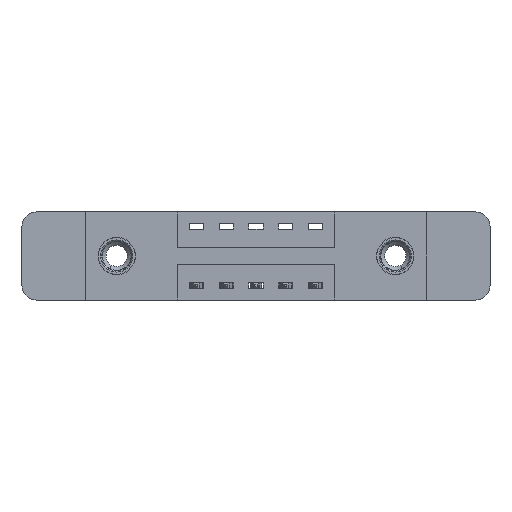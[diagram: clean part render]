
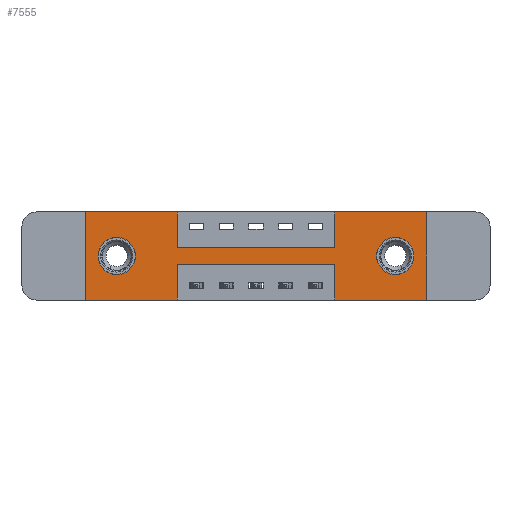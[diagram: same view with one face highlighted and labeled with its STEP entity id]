
A CAD part, front view. The second image highlights one B-rep face of the part: STEP entity #7555.
In plain terms, the highlighted planar face has unit normal (0, -1, 0).
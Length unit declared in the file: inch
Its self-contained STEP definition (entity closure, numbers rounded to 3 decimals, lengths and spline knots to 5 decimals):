
#7 = EDGE_CURVE ( 'NONE', #7786, #2454, #1814, .T. ) ;
#80 = CARTESIAN_POINT ( 'NONE',  ( 0.3875, 0., -0.15 ) ) ;
#185 = EDGE_CURVE ( 'NONE', #9656, #5307, #685, .T. ) ;
#569 = DIRECTION ( 'NONE',  ( 0., 0., -1. ) ) ;
#576 = CARTESIAN_POINT ( 'NONE',  ( 1.435, 0., -0.37 ) ) ;
#598 = DIRECTION ( 'NONE',  ( 1., 0., 0. ) ) ;
#685 = CIRCLE ( 'NONE', #3351, 0.078 ) ;
#688 = CARTESIAN_POINT ( 'NONE',  ( 1.3025, 0., -0.107 ) ) ;
#735 = CARTESIAN_POINT ( 'NONE',  ( 1.0475, 0., -0.15 ) ) ;
#748 = EDGE_CURVE ( 'NONE', #1055, #12500, #4042, .T. ) ;
#827 = EDGE_CURVE ( 'NONE', #8503, #7786, #8581, .T. ) ;
#932 = ORIENTED_EDGE ( 'NONE', *, *, #4530, .F. ) ;
#994 = CARTESIAN_POINT ( 'NONE',  ( 0., 0., 0. ) ) ;
#1055 = VERTEX_POINT ( 'NONE', #735 ) ;
#1070 = EDGE_LOOP ( 'NONE', ( #12165, #3451 ) ) ;
#1083 = EDGE_CURVE ( 'NONE', #12500, #12833, #3960, .T. ) ;
#1120 = CARTESIAN_POINT ( 'NONE',  ( 1.3025, 0., -0.185 ) ) ;
#1148 = DIRECTION ( 'NONE',  ( -1., 0., 0. ) ) ;
#1228 = VERTEX_POINT ( 'NONE', #576 ) ;
#1241 = ORIENTED_EDGE ( 'NONE', *, *, #9918, .F. ) ;
#1318 = CARTESIAN_POINT ( 'NONE',  ( 0.3875, 0., 0. ) ) ;
#1526 = EDGE_CURVE ( 'NONE', #2454, #10739, #7697, .T. ) ;
#1574 = DIRECTION ( 'NONE',  ( 0., 0., 1. ) ) ;
#1666 = FACE_BOUND ( 'NONE', #1070, .T. ) ;
#1814 = LINE ( 'NONE', #994, #6678 ) ;
#1844 = VECTOR ( 'NONE', #8648, 39.37008 ) ;
#1869 = CARTESIAN_POINT ( 'NONE',  ( 1.0475, 0., 0. ) ) ;
#1933 = EDGE_CURVE ( 'NONE', #12833, #1228, #7547, .T. ) ;
#1997 = CARTESIAN_POINT ( 'NONE',  ( 0.1325, 0., -0.263 ) ) ;
#2264 = DIRECTION ( 'NONE',  ( 0., 0., -1. ) ) ;
#2392 = EDGE_CURVE ( 'NONE', #12311, #5553, #10341, .T. ) ;
#2421 = EDGE_CURVE ( 'NONE', #5553, #12311, #3495, .T. ) ;
#2454 = VERTEX_POINT ( 'NONE', #4477 ) ;
#2648 = CARTESIAN_POINT ( 'NONE',  ( 0.3875, 0., -0.37 ) ) ;
#2805 = DIRECTION ( 'NONE',  ( 0., 0., -1. ) ) ;
#2867 = DIRECTION ( 'NONE',  ( 0., 0., 1. ) ) ;
#3082 = DIRECTION ( 'NONE',  ( 0., 0., -1. ) ) ;
#3159 = CARTESIAN_POINT ( 'NONE',  ( 1.3025, 0., -0.263 ) ) ;
#3272 = VERTEX_POINT ( 'NONE', #5117 ) ;
#3351 = AXIS2_PLACEMENT_3D ( 'NONE', #8488, #3353, #7647 ) ;
#3353 = DIRECTION ( 'NONE',  ( 0., 1., 0. ) ) ;
#3428 = DIRECTION ( 'NONE',  ( 0., 0., -1. ) ) ;
#3451 = ORIENTED_EDGE ( 'NONE', *, *, #12681, .T. ) ;
#3495 = CIRCLE ( 'NONE', #12816, 0.078 ) ;
#3581 = ORIENTED_EDGE ( 'NONE', *, *, #1933, .F. ) ;
#3729 = VERTEX_POINT ( 'NONE', #5995 ) ;
#3768 = FACE_BOUND ( 'NONE', #7127, .T. ) ;
#3927 = CARTESIAN_POINT ( 'NONE',  ( 0.1325, 0., -0.107 ) ) ;
#3960 = LINE ( 'NONE', #6140, #5457 ) ;
#3982 = ORIENTED_EDGE ( 'NONE', *, *, #748, .F. ) ;
#4029 = DIRECTION ( 'NONE',  ( -1., 0., 0. ) ) ;
#4042 = LINE ( 'NONE', #10263, #10501 ) ;
#4073 = DIRECTION ( 'NONE',  ( 1., 0., 0. ) ) ;
#4165 = CARTESIAN_POINT ( 'NONE',  ( 1.435, 0., 0. ) ) ;
#4201 = DIRECTION ( 'NONE',  ( 0., 0., -1. ) ) ;
#4278 = EDGE_CURVE ( 'NONE', #3729, #3272, #6508, .T. ) ;
#4341 = AXIS2_PLACEMENT_3D ( 'NONE', #12305, #9233, #2805 ) ;
#4477 = CARTESIAN_POINT ( 'NONE',  ( 0.3875, 0., 0. ) ) ;
#4530 = EDGE_CURVE ( 'NONE', #1228, #3729, #12153, .T. ) ;
#5050 = VECTOR ( 'NONE', #3428, 39.37008 ) ;
#5063 = DIRECTION ( 'NONE',  ( 0., 1., 0. ) ) ;
#5117 = CARTESIAN_POINT ( 'NONE',  ( 1.0475, 0., -0.22 ) ) ;
#5216 = EDGE_LOOP ( 'NONE', ( #11760, #1241, #5515, #932, #3581, #10585, #3982, #10959, #8956, #6202, #7494, #9322 ) ) ;
#5307 = VERTEX_POINT ( 'NONE', #1997 ) ;
#5457 = VECTOR ( 'NONE', #598, 39.37008 ) ;
#5515 = ORIENTED_EDGE ( 'NONE', *, *, #4278, .F. ) ;
#5553 = VERTEX_POINT ( 'NONE', #3159 ) ;
#5995 = CARTESIAN_POINT ( 'NONE',  ( 1.0475, 0., -0.37 ) ) ;
#6140 = CARTESIAN_POINT ( 'NONE',  ( 0., 0., 0. ) ) ;
#6202 = ORIENTED_EDGE ( 'NONE', *, *, #7, .F. ) ;
#6413 = DIRECTION ( 'NONE',  ( 0., 1., 0. ) ) ;
#6508 = LINE ( 'NONE', #9690, #10647 ) ;
#6565 = CARTESIAN_POINT ( 'NONE',  ( 0., 0., 0. ) ) ;
#6678 = VECTOR ( 'NONE', #4073, 39.37008 ) ;
#6757 = DIRECTION ( 'NONE',  ( -1., 0., 0. ) ) ;
#7127 = EDGE_LOOP ( 'NONE', ( #9303, #12239 ) ) ;
#7134 = LINE ( 'NONE', #11383, #12633 ) ;
#7238 = AXIS2_PLACEMENT_3D ( 'NONE', #11670, #6413, #4201 ) ;
#7291 = CARTESIAN_POINT ( 'NONE',  ( 0.3875, 0., -0.15 ) ) ;
#7494 = ORIENTED_EDGE ( 'NONE', *, *, #827, .F. ) ;
#7547 = LINE ( 'NONE', #11774, #11883 ) ;
#7555 = ADVANCED_FACE ( 'NONE', ( #3768, #1666, #10268 ), #9089, .T. ) ;
#7647 = DIRECTION ( 'NONE',  ( 0., 0., 1. ) ) ;
#7671 = DIRECTION ( 'NONE',  ( 0., 0., 1. ) ) ;
#7697 = LINE ( 'NONE', #1318, #5050 ) ;
#7786 = VERTEX_POINT ( 'NONE', #6565 ) ;
#7936 = VECTOR ( 'NONE', #6757, 39.37008 ) ;
#8050 = VERTEX_POINT ( 'NONE', #13691 ) ;
#8488 = CARTESIAN_POINT ( 'NONE',  ( 0.1325, 0., -0.185 ) ) ;
#8503 = VERTEX_POINT ( 'NONE', #13422 ) ;
#8507 = CARTESIAN_POINT ( 'NONE',  ( 0., 0., -0.37 ) ) ;
#8581 = LINE ( 'NONE', #10750, #1844 ) ;
#8648 = DIRECTION ( 'NONE',  ( 0., 0., 1. ) ) ;
#8956 = ORIENTED_EDGE ( 'NONE', *, *, #1526, .F. ) ;
#9079 = EDGE_CURVE ( 'NONE', #10739, #1055, #12674, .T. ) ;
#9089 = PLANE ( 'NONE',  #4341 ) ;
#9233 = DIRECTION ( 'NONE',  ( 0., -1., 0. ) ) ;
#9303 = ORIENTED_EDGE ( 'NONE', *, *, #2392, .T. ) ;
#9322 = ORIENTED_EDGE ( 'NONE', *, *, #12462, .F. ) ;
#9566 = VECTOR ( 'NONE', #1148, 39.37008 ) ;
#9626 = VECTOR ( 'NONE', #11547, 39.37008 ) ;
#9656 = VERTEX_POINT ( 'NONE', #3927 ) ;
#9690 = CARTESIAN_POINT ( 'NONE',  ( 1.0475, 0., -0.37 ) ) ;
#9918 = EDGE_CURVE ( 'NONE', #3272, #8050, #7134, .T. ) ;
#10263 = CARTESIAN_POINT ( 'NONE',  ( 1.0475, 0., 0. ) ) ;
#10268 = FACE_OUTER_BOUND ( 'NONE', #5216, .T. ) ;
#10341 = CIRCLE ( 'NONE', #7238, 0.078 ) ;
#10501 = VECTOR ( 'NONE', #2867, 39.37008 ) ;
#10585 = ORIENTED_EDGE ( 'NONE', *, *, #1083, .F. ) ;
#10586 = LINE ( 'NONE', #8507, #9566 ) ;
#10647 = VECTOR ( 'NONE', #7671, 39.37008 ) ;
#10739 = VERTEX_POINT ( 'NONE', #80 ) ;
#10750 = CARTESIAN_POINT ( 'NONE',  ( 0., 0., 0. ) ) ;
#10959 = ORIENTED_EDGE ( 'NONE', *, *, #9079, .F. ) ;
#11097 = CARTESIAN_POINT ( 'NONE',  ( 0., 0., -0.37 ) ) ;
#11153 = VERTEX_POINT ( 'NONE', #12582 ) ;
#11241 = CARTESIAN_POINT ( 'NONE',  ( 0.1325, 0., -0.185 ) ) ;
#11383 = CARTESIAN_POINT ( 'NONE',  ( 0.3875, 0., -0.22 ) ) ;
#11446 = EDGE_CURVE ( 'NONE', #8050, #11153, #13211, .T. ) ;
#11547 = DIRECTION ( 'NONE',  ( 1., 0., 0. ) ) ;
#11584 = CIRCLE ( 'NONE', #13125, 0.078 ) ;
#11586 = VECTOR ( 'NONE', #569, 39.37008 ) ;
#11670 = CARTESIAN_POINT ( 'NONE',  ( 1.3025, 0., -0.185 ) ) ;
#11760 = ORIENTED_EDGE ( 'NONE', *, *, #11446, .F. ) ;
#11774 = CARTESIAN_POINT ( 'NONE',  ( 1.435, 0., 0. ) ) ;
#11883 = VECTOR ( 'NONE', #2264, 39.37008 ) ;
#12153 = LINE ( 'NONE', #11097, #7936 ) ;
#12165 = ORIENTED_EDGE ( 'NONE', *, *, #185, .T. ) ;
#12239 = ORIENTED_EDGE ( 'NONE', *, *, #2421, .T. ) ;
#12305 = CARTESIAN_POINT ( 'NONE',  ( 0., 0., -0.37 ) ) ;
#12311 = VERTEX_POINT ( 'NONE', #688 ) ;
#12462 = EDGE_CURVE ( 'NONE', #11153, #8503, #10586, .T. ) ;
#12500 = VERTEX_POINT ( 'NONE', #1869 ) ;
#12582 = CARTESIAN_POINT ( 'NONE',  ( 0.3875, 0., -0.37 ) ) ;
#12633 = VECTOR ( 'NONE', #4029, 39.37008 ) ;
#12674 = LINE ( 'NONE', #7291, #9626 ) ;
#12675 = DIRECTION ( 'NONE',  ( 0., 1., 0. ) ) ;
#12681 = EDGE_CURVE ( 'NONE', #5307, #9656, #11584, .T. ) ;
#12816 = AXIS2_PLACEMENT_3D ( 'NONE', #1120, #12675, #3082 ) ;
#12833 = VERTEX_POINT ( 'NONE', #4165 ) ;
#13125 = AXIS2_PLACEMENT_3D ( 'NONE', #11241, #5063, #1574 ) ;
#13211 = LINE ( 'NONE', #2648, #11586 ) ;
#13422 = CARTESIAN_POINT ( 'NONE',  ( 0., 0., -0.37 ) ) ;
#13691 = CARTESIAN_POINT ( 'NONE',  ( 0.3875, 0., -0.22 ) ) ;
